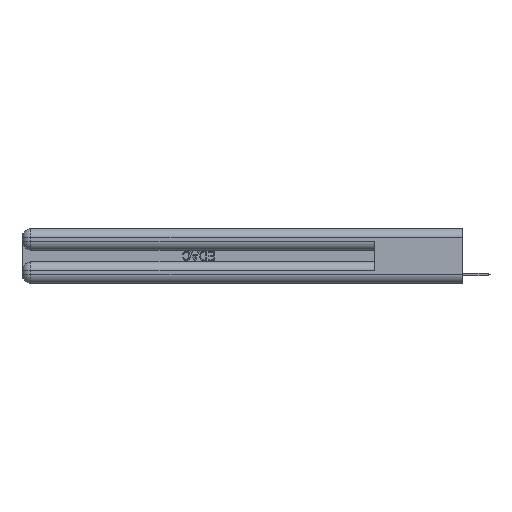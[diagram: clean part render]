
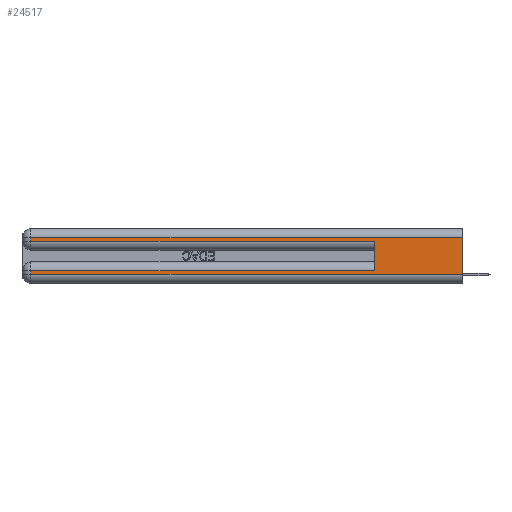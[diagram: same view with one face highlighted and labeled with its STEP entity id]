
A CAD part, left-side view. The second image highlights one B-rep face of the part: STEP entity #24517.
In plain terms, the highlighted planar face has unit normal (-1, 0, 0).
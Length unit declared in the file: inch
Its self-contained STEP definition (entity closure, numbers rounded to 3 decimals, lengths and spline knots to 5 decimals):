
#94 = VERTEX_POINT ( 'NONE', #16919 ) ;
#586 = LINE ( 'NONE', #21043, #3857 ) ;
#1578 = LINE ( 'NONE', #16725, #7064 ) ;
#2560 = ORIENTED_EDGE ( 'NONE', *, *, #24995, .T. ) ;
#2577 = VERTEX_POINT ( 'NONE', #9963 ) ;
#3624 = ORIENTED_EDGE ( 'NONE', *, *, #26922, .T. ) ;
#3857 = VECTOR ( 'NONE', #9232, 39.37008 ) ;
#4290 = DIRECTION ( 'NONE',  ( 0., 1., 0. ) ) ;
#4483 = ORIENTED_EDGE ( 'NONE', *, *, #10403, .T. ) ;
#4830 = DIRECTION ( 'NONE',  ( 0., -1., 0. ) ) ;
#4977 = VECTOR ( 'NONE', #11212, 39.37008 ) ;
#5105 = DIRECTION ( 'NONE',  ( 0., 0., -1. ) ) ;
#5122 = CARTESIAN_POINT ( 'NONE',  ( 0., 0., 0.06 ) ) ;
#5221 = VERTEX_POINT ( 'NONE', #21908 ) ;
#5423 = ORIENTED_EDGE ( 'NONE', *, *, #12965, .F. ) ;
#5467 = ORIENTED_EDGE ( 'NONE', *, *, #7378, .T. ) ;
#5785 = CARTESIAN_POINT ( 'NONE',  ( 0., 0.6, 0.145 ) ) ;
#6028 = VECTOR ( 'NONE', #26866, 39.37008 ) ;
#6557 = LINE ( 'NONE', #29832, #25322 ) ;
#7064 = VECTOR ( 'NONE', #5105, 39.37008 ) ;
#7097 = VECTOR ( 'NONE', #4830, 39.37008 ) ;
#7378 = EDGE_CURVE ( 'NONE', #2577, #94, #586, .T. ) ;
#7625 = EDGE_CURVE ( 'NONE', #21309, #5221, #11947, .T. ) ;
#7934 = VECTOR ( 'NONE', #16573, 39.37008 ) ;
#9055 = VERTEX_POINT ( 'NONE', #20861 ) ;
#9232 = DIRECTION ( 'NONE',  ( 0., 0., -1. ) ) ;
#9294 = DIRECTION ( 'NONE',  ( 1., 0., 0. ) ) ;
#9963 = CARTESIAN_POINT ( 'NONE',  ( 0., 2.94, 0.085 ) ) ;
#10403 = EDGE_CURVE ( 'NONE', #94, #16633, #6557, .T. ) ;
#11212 = DIRECTION ( 'NONE',  ( 0., 1., 0. ) ) ;
#11573 = LINE ( 'NONE', #20240, #4977 ) ;
#11832 = DIRECTION ( 'NONE',  ( 0., -1., 0. ) ) ;
#11947 = LINE ( 'NONE', #20917, #7934 ) ;
#12597 = EDGE_CURVE ( 'NONE', #23701, #21309, #11573, .T. ) ;
#12965 = EDGE_CURVE ( 'NONE', #9055, #24922, #15620, .T. ) ;
#13396 = FACE_OUTER_BOUND ( 'NONE', #24525, .T. ) ;
#14088 = DIRECTION ( 'NONE',  ( 0., 0., -1. ) ) ;
#15620 = LINE ( 'NONE', #5785, #6028 ) ;
#16502 = ORIENTED_EDGE ( 'NONE', *, *, #18760, .F. ) ;
#16573 = DIRECTION ( 'NONE',  ( 0., 0., -1. ) ) ;
#16633 = VERTEX_POINT ( 'NONE', #5122 ) ;
#16725 = CARTESIAN_POINT ( 'NONE',  ( 0., 0., 0.37 ) ) ;
#16919 = CARTESIAN_POINT ( 'NONE',  ( 0., 2.94, 0.06 ) ) ;
#17880 = AXIS2_PLACEMENT_3D ( 'NONE', #27794, #9294, #14088 ) ;
#18323 = CARTESIAN_POINT ( 'NONE',  ( 0., 0.6, 0.285 ) ) ;
#18760 = EDGE_CURVE ( 'NONE', #23701, #16633, #1578, .T. ) ;
#20240 = CARTESIAN_POINT ( 'NONE',  ( 0., 0., 0.31 ) ) ;
#20316 = LINE ( 'NONE', #29873, #29851 ) ;
#20861 = CARTESIAN_POINT ( 'NONE',  ( 0., 0.6, 0.085 ) ) ;
#20917 = CARTESIAN_POINT ( 'NONE',  ( 0., 2.94, 0.37 ) ) ;
#21043 = CARTESIAN_POINT ( 'NONE',  ( 0., 2.94, 0.37 ) ) ;
#21309 = VERTEX_POINT ( 'NONE', #25239 ) ;
#21908 = CARTESIAN_POINT ( 'NONE',  ( 0., 2.94, 0.285 ) ) ;
#22160 = CARTESIAN_POINT ( 'NONE',  ( 0., 0., 0.31 ) ) ;
#23701 = VERTEX_POINT ( 'NONE', #22160 ) ;
#24517 = ADVANCED_FACE ( 'NONE', ( #13396 ), #25417, .F. ) ;
#24525 = EDGE_LOOP ( 'NONE', ( #16502, #30105, #25979, #2560, #5423, #3624, #5467, #4483 ) ) ;
#24922 = VERTEX_POINT ( 'NONE', #18323 ) ;
#24995 = EDGE_CURVE ( 'NONE', #5221, #24922, #29168, .T. ) ;
#25239 = CARTESIAN_POINT ( 'NONE',  ( 0., 2.94, 0.31 ) ) ;
#25322 = VECTOR ( 'NONE', #11832, 39.37008 ) ;
#25417 = PLANE ( 'NONE',  #17880 ) ;
#25783 = CARTESIAN_POINT ( 'NONE',  ( 0., 0., 0.285 ) ) ;
#25979 = ORIENTED_EDGE ( 'NONE', *, *, #7625, .T. ) ;
#26866 = DIRECTION ( 'NONE',  ( 0., 0., 1. ) ) ;
#26922 = EDGE_CURVE ( 'NONE', #9055, #2577, #20316, .T. ) ;
#27794 = CARTESIAN_POINT ( 'NONE',  ( 0., 0., 0.37 ) ) ;
#29168 = LINE ( 'NONE', #25783, #7097 ) ;
#29832 = CARTESIAN_POINT ( 'NONE',  ( 0., 0., 0.06 ) ) ;
#29851 = VECTOR ( 'NONE', #4290, 39.37008 ) ;
#29873 = CARTESIAN_POINT ( 'NONE',  ( 0., 0., 0.085 ) ) ;
#30105 = ORIENTED_EDGE ( 'NONE', *, *, #12597, .T. ) ;
